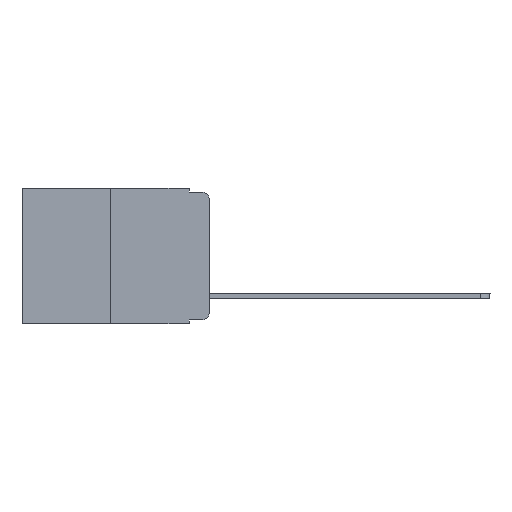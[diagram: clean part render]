
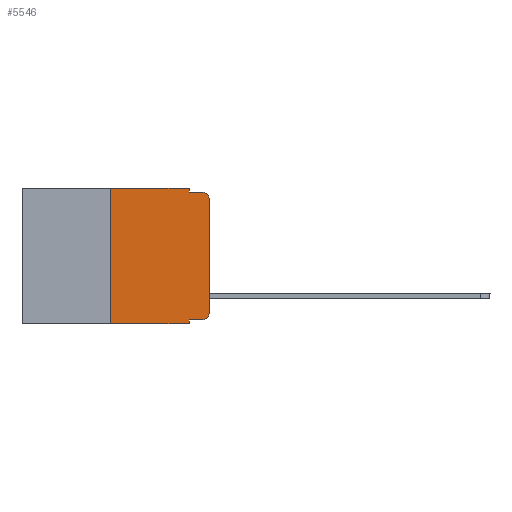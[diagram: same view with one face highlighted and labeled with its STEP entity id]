
A CAD part, left-side view. The second image highlights one B-rep face of the part: STEP entity #5546.
In plain terms, the highlighted planar face has unit normal (-1, 0, 0).
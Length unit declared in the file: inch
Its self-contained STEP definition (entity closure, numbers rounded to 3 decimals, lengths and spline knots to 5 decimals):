
#384 = AXIS2_PLACEMENT_3D ( 'NONE', #8854, #3224, #16207 ) ;
#1003 = LINE ( 'NONE', #3221, #12909 ) ;
#1696 = PLANE ( 'NONE',  #2987 ) ;
#2847 = ORIENTED_EDGE ( 'NONE', *, *, #8454, .F. ) ;
#2987 = AXIS2_PLACEMENT_3D ( 'NONE', #20235, #3903, #7106 ) ;
#3209 = VECTOR ( 'NONE', #5508, 39.37008 ) ;
#3221 = CARTESIAN_POINT ( 'NONE',  ( 0., 0.051, -0.333 ) ) ;
#3224 = DIRECTION ( 'NONE',  ( -1., 0., 0. ) ) ;
#3443 = ORIENTED_EDGE ( 'NONE', *, *, #11346, .F. ) ;
#3557 = LINE ( 'NONE', #24032, #8531 ) ;
#3903 = DIRECTION ( 'NONE',  ( 1., 0., 0. ) ) ;
#4073 = DIRECTION ( 'NONE',  ( 0., -1., 0. ) ) ;
#5051 = VERTEX_POINT ( 'NONE', #20264 ) ;
#5508 = DIRECTION ( 'NONE',  ( 0., -1., 0. ) ) ;
#5546 = ADVANCED_FACE ( 'NONE', ( #20705 ), #1696, .F. ) ;
#5614 = CARTESIAN_POINT ( 'NONE',  ( 0., 0.473, 0. ) ) ;
#6018 = VECTOR ( 'NONE', #9256, 39.37008 ) ;
#6238 = LINE ( 'NONE', #10142, #6561 ) ;
#6561 = VECTOR ( 'NONE', #20948, 39.37008 ) ;
#6908 = ORIENTED_EDGE ( 'NONE', *, *, #7789, .F. ) ;
#6924 = DIRECTION ( 'NONE',  ( 0., 0., 1. ) ) ;
#7080 = CARTESIAN_POINT ( 'NONE',  ( 0., 0.051, 0. ) ) ;
#7096 = CARTESIAN_POINT ( 'NONE',  ( 0., 0.25, 0. ) ) ;
#7100 = EDGE_LOOP ( 'NONE', ( #16771, #13168, #6908, #2847, #17264, #21655, #19099, #3443, #16467, #22196 ) ) ;
#7106 = DIRECTION ( 'NONE',  ( 0., 0., -1. ) ) ;
#7365 = VERTEX_POINT ( 'NONE', #16976 ) ;
#7556 = EDGE_CURVE ( 'NONE', #15655, #19650, #10586, .T. ) ;
#7789 = EDGE_CURVE ( 'NONE', #17332, #15148, #9584, .T. ) ;
#7861 = VECTOR ( 'NONE', #4073, 39.37008 ) ;
#8454 = EDGE_CURVE ( 'NONE', #5051, #17332, #3557, .T. ) ;
#8531 = VECTOR ( 'NONE', #16168, 39.37008 ) ;
#8601 = CIRCLE ( 'NONE', #384, 0.02 ) ;
#8613 = DIRECTION ( 'NONE',  ( 0., -1., 0. ) ) ;
#8854 = CARTESIAN_POINT ( 'NONE',  ( 0., 0.02, -0.03 ) ) ;
#9024 = LINE ( 'NONE', #7080, #6018 ) ;
#9256 = DIRECTION ( 'NONE',  ( 0., 0., -1. ) ) ;
#9399 = LINE ( 'NONE', #5614, #3209 ) ;
#9521 = EDGE_CURVE ( 'NONE', #19650, #5051, #9399, .T. ) ;
#9584 = LINE ( 'NONE', #17063, #7861 ) ;
#9977 = VERTEX_POINT ( 'NONE', #12935 ) ;
#10142 = CARTESIAN_POINT ( 'NONE',  ( 0., 0.473, -0.343 ) ) ;
#10586 = LINE ( 'NONE', #23727, #19981 ) ;
#11346 = EDGE_CURVE ( 'NONE', #7365, #21249, #9024, .T. ) ;
#11690 = AXIS2_PLACEMENT_3D ( 'NONE', #20373, #21697, #23920 ) ;
#12909 = VECTOR ( 'NONE', #8613, 39.37008 ) ;
#12935 = CARTESIAN_POINT ( 'NONE',  ( 0., 0.02, -0.333 ) ) ;
#13168 = ORIENTED_EDGE ( 'NONE', *, *, #20394, .T. ) ;
#14165 = CARTESIAN_POINT ( 'NONE',  ( 0., 0.051, -0.343 ) ) ;
#15148 = VERTEX_POINT ( 'NONE', #23663 ) ;
#15312 = CARTESIAN_POINT ( 'NONE',  ( 0., 0., -0.03 ) ) ;
#15655 = VERTEX_POINT ( 'NONE', #23892 ) ;
#16120 = VERTEX_POINT ( 'NONE', #15312 ) ;
#16168 = DIRECTION ( 'NONE',  ( 0., 0., -1. ) ) ;
#16207 = DIRECTION ( 'NONE',  ( 0., 0., -1. ) ) ;
#16380 = VECTOR ( 'NONE', #6924, 39.37008 ) ;
#16467 = ORIENTED_EDGE ( 'NONE', *, *, #19109, .T. ) ;
#16591 = DIRECTION ( 'NONE',  ( 0., 0., 1. ) ) ;
#16698 = EDGE_CURVE ( 'NONE', #15655, #21249, #6238, .T. ) ;
#16771 = ORIENTED_EDGE ( 'NONE', *, *, #17397, .T. ) ;
#16976 = CARTESIAN_POINT ( 'NONE',  ( 0., 0.051, -0.333 ) ) ;
#17063 = CARTESIAN_POINT ( 'NONE',  ( 0., 0.051, -0.01 ) ) ;
#17182 = CIRCLE ( 'NONE', #11690, 0.02 ) ;
#17264 = ORIENTED_EDGE ( 'NONE', *, *, #9521, .F. ) ;
#17332 = VERTEX_POINT ( 'NONE', #22881 ) ;
#17397 = EDGE_CURVE ( 'NONE', #19909, #16120, #21523, .T. ) ;
#17694 = CARTESIAN_POINT ( 'NONE',  ( 0., 0., 0. ) ) ;
#17940 = EDGE_CURVE ( 'NONE', #9977, #19909, #17182, .T. ) ;
#19099 = ORIENTED_EDGE ( 'NONE', *, *, #16698, .T. ) ;
#19109 = EDGE_CURVE ( 'NONE', #7365, #9977, #1003, .T. ) ;
#19650 = VERTEX_POINT ( 'NONE', #7096 ) ;
#19909 = VERTEX_POINT ( 'NONE', #23136 ) ;
#19981 = VECTOR ( 'NONE', #16591, 39.37008 ) ;
#20235 = CARTESIAN_POINT ( 'NONE',  ( 0., 0.473, 0. ) ) ;
#20264 = CARTESIAN_POINT ( 'NONE',  ( 0., 0.051, 0. ) ) ;
#20373 = CARTESIAN_POINT ( 'NONE',  ( 0., 0.02, -0.313 ) ) ;
#20394 = EDGE_CURVE ( 'NONE', #16120, #15148, #8601, .T. ) ;
#20705 = FACE_OUTER_BOUND ( 'NONE', #7100, .T. ) ;
#20948 = DIRECTION ( 'NONE',  ( 0., -1., 0. ) ) ;
#21249 = VERTEX_POINT ( 'NONE', #14165 ) ;
#21523 = LINE ( 'NONE', #17694, #16380 ) ;
#21655 = ORIENTED_EDGE ( 'NONE', *, *, #7556, .F. ) ;
#21697 = DIRECTION ( 'NONE',  ( -1., 0., 0. ) ) ;
#22196 = ORIENTED_EDGE ( 'NONE', *, *, #17940, .T. ) ;
#22881 = CARTESIAN_POINT ( 'NONE',  ( 0., 0.051, -0.01 ) ) ;
#23136 = CARTESIAN_POINT ( 'NONE',  ( 0., 0., -0.313 ) ) ;
#23663 = CARTESIAN_POINT ( 'NONE',  ( 0., 0.02, -0.01 ) ) ;
#23727 = CARTESIAN_POINT ( 'NONE',  ( 0., 0.25, 0. ) ) ;
#23892 = CARTESIAN_POINT ( 'NONE',  ( 0., 0.25, -0.343 ) ) ;
#23920 = DIRECTION ( 'NONE',  ( 0., 0., -1. ) ) ;
#24032 = CARTESIAN_POINT ( 'NONE',  ( 0., 0.051, 0. ) ) ;
